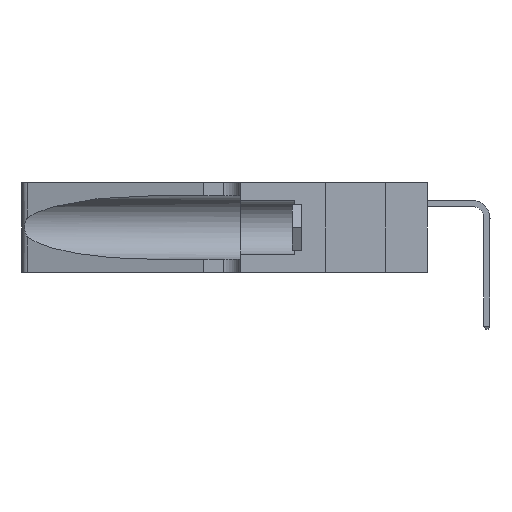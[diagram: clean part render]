
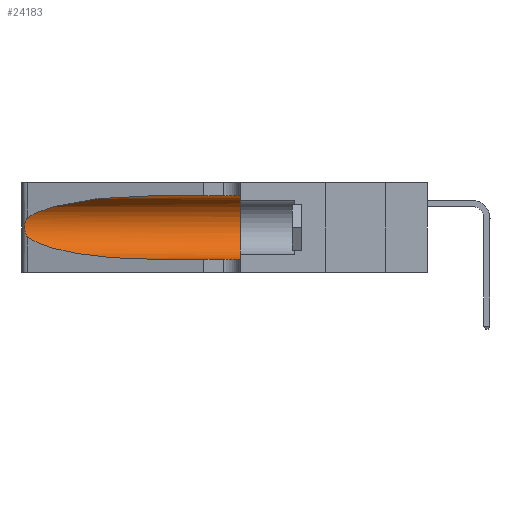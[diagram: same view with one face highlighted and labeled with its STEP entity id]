
A CAD part, left-side view. The second image highlights one B-rep face of the part: STEP entity #24183.
In plain terms, the highlighted cylindrical face has radius 3.308 mm (diameter 6.617 mm), a partial arc.
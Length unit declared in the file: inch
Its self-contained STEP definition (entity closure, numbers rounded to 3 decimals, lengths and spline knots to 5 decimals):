
#430 = CARTESIAN_POINT ( 'NONE',  ( 0.25787, 1.23484, 0.2124 ) ) ;
#478 = CARTESIAN_POINT ( 'NONE',  ( 0.25854, 1.2359, 0.20912 ) ) ;
#664 = CARTESIAN_POINT ( 'NONE',  ( 0.25639, 1.23184, 0.21858 ) ) ;
#1391 = EDGE_LOOP ( 'NONE', ( #30946, #7297, #7504, #7036, #8586, #23628 ) ) ;
#3697 = VERTEX_POINT ( 'NONE', #26931 ) ;
#4834 = EDGE_CURVE ( 'NONE', #18906, #3697, #22312, .T. ) ;
#5140 = CARTESIAN_POINT ( 'NONE',  ( 0.26018, 1.23835, 0.19895 ) ) ;
#5648 = EDGE_CURVE ( 'NONE', #36253, #10619, #7932, .T. ) ;
#7036 = ORIENTED_EDGE ( 'NONE', *, *, #29105, .T. ) ;
#7297 = ORIENTED_EDGE ( 'NONE', *, *, #25240, .T. ) ;
#7504 = ORIENTED_EDGE ( 'NONE', *, *, #5648, .T. ) ;
#7932 =( BOUNDED_CURVE ( )  B_SPLINE_CURVE ( 3, ( #16820, #29108, #18029, #36626 ),
 .UNSPECIFIED., .F., .T. ) 
 B_SPLINE_CURVE_WITH_KNOTS ( ( 4, 4 ),
 ( 3.44316, 4.71239 ),
 .UNSPECIFIED. ) 
 CURVE ( )  GEOMETRIC_REPRESENTATION_ITEM ( )  RATIONAL_B_SPLINE_CURVE ( ( 1., 0.87, 0.87, 1. ) ) 
 REPRESENTATION_ITEM ( '' )  );
#8586 = ORIENTED_EDGE ( 'NONE', *, *, #4834, .F. ) ;
#8799 = CARTESIAN_POINT ( 'NONE',  ( 0.25487, 1.22718, 0.14631 ) ) ;
#9832 = AXIS2_PLACEMENT_3D ( 'NONE', #17270, #25942, #23072 ) ;
#10583 = CARTESIAN_POINT ( 'NONE',  ( 0.1305, 0.72297, 0.31525 ) ) ;
#10619 = VERTEX_POINT ( 'NONE', #29680 ) ;
#10763 = CARTESIAN_POINT ( 'NONE',  ( 0.1305, 1.61858, 0.31525 ) ) ;
#12859 = CARTESIAN_POINT ( 'NONE',  ( 0.25487, 1.22718, 0.22369 ) ) ;
#12988 = CARTESIAN_POINT ( 'NONE',  ( 0.2373, 1.15595, 0.28018 ) ) ;
#13451 = LINE ( 'NONE', #10763, #23285 ) ;
#13997 =( BOUNDED_CURVE ( )  B_SPLINE_CURVE ( 3, ( #24411, #27498, #12988, #33497 ),
 .UNSPECIFIED., .F., .T. ) 
 B_SPLINE_CURVE_WITH_KNOTS ( ( 4, 4 ),
 ( 1.5708, 2.84003 ),
 .UNSPECIFIED. ) 
 CURVE ( )  GEOMETRIC_REPRESENTATION_ITEM ( )  RATIONAL_B_SPLINE_CURVE ( ( 1., 0.87, 0.87, 1. ) ) 
 REPRESENTATION_ITEM ( '' )  );
#14164 = FACE_OUTER_BOUND ( 'NONE', #1391, .T. ) ;
#14249 = VERTEX_POINT ( 'NONE', #10583 ) ;
#15448 = CYLINDRICAL_SURFACE ( 'NONE', #9832, 0.13025 ) ;
#16820 = CARTESIAN_POINT ( 'NONE',  ( 0.25487, 1.22718, 0.14631 ) ) ;
#17270 = CARTESIAN_POINT ( 'NONE',  ( 0.1305, 1.61858, 0.185 ) ) ;
#17485 = VECTOR ( 'NONE', #26968, 39.37008 ) ;
#17696 = LINE ( 'NONE', #24034, #17485 ) ;
#17855 = EDGE_CURVE ( 'NONE', #14249, #18906, #13451, .T. ) ;
#18029 = CARTESIAN_POINT ( 'NONE',  ( 0.18966, 0.96281, 0.05475 ) ) ;
#18906 = VERTEX_POINT ( 'NONE', #31943 ) ;
#19440 = DIRECTION ( 'NONE',  ( 0., -1., 0. ) ) ;
#20241 = VERTEX_POINT ( 'NONE', #12859 ) ;
#22207 = CARTESIAN_POINT ( 'NONE',  ( 0.1305, 0.35, 0.185 ) ) ;
#22312 = CIRCLE ( 'NONE', #26788, 0.13025 ) ;
#23072 = DIRECTION ( 'NONE',  ( 0., 0., -1. ) ) ;
#23285 = VECTOR ( 'NONE', #19440, 39.37008 ) ;
#23628 = ORIENTED_EDGE ( 'NONE', *, *, #17855, .F. ) ;
#24034 = CARTESIAN_POINT ( 'NONE',  ( 0.1305, 1.61858, 0.05475 ) ) ;
#24183 = ADVANCED_FACE ( 'NONE', ( #14164 ), #15448, .F. ) ;
#24411 = CARTESIAN_POINT ( 'NONE',  ( 0.1305, 0.72297, 0.31525 ) ) ;
#25240 = EDGE_CURVE ( 'NONE', #20241, #36253, #27399, .T. ) ;
#25670 = DIRECTION ( 'NONE',  ( 0., 0., 1. ) ) ;
#25942 = DIRECTION ( 'NONE',  ( 0., -1., 0. ) ) ;
#26788 = AXIS2_PLACEMENT_3D ( 'NONE', #22207, #36296, #25670 ) ;
#26931 = CARTESIAN_POINT ( 'NONE',  ( 0.1305, 0.35, 0.05475 ) ) ;
#26968 = DIRECTION ( 'NONE',  ( 0., -1., 0. ) ) ;
#27399 = B_SPLINE_CURVE_WITH_KNOTS ( 'NONE', 3,
 ( #37388, #37234, #664, #430, #478, #5140, #27731, #27726, #27646, #28073, #28239, #28335, #27817, #27683 ),
 .UNSPECIFIED., .F., .F.,
 ( 4, 2, 2, 2, 2, 2, 4 ),
 ( 0., 0.00027, 0.00053, 0.00107, 0.0016, 0.00187, 0.00214 ),
 .UNSPECIFIED. ) ;
#27498 = CARTESIAN_POINT ( 'NONE',  ( 0.18966, 0.96281, 0.31525 ) ) ;
#27646 = CARTESIAN_POINT ( 'NONE',  ( 0.26017, 1.23833, 0.17102 ) ) ;
#27683 = CARTESIAN_POINT ( 'NONE',  ( 0.25487, 1.22718, 0.14631 ) ) ;
#27726 = CARTESIAN_POINT ( 'NONE',  ( 0.26075, 1.23896, 0.178 ) ) ;
#27731 = CARTESIAN_POINT ( 'NONE',  ( 0.26075, 1.23896, 0.19203 ) ) ;
#27817 = CARTESIAN_POINT ( 'NONE',  ( 0.25555, 1.22993, 0.14849 ) ) ;
#28073 = CARTESIAN_POINT ( 'NONE',  ( 0.25856, 1.23593, 0.16098 ) ) ;
#28239 = CARTESIAN_POINT ( 'NONE',  ( 0.25789, 1.23486, 0.15765 ) ) ;
#28335 = CARTESIAN_POINT ( 'NONE',  ( 0.25639, 1.23186, 0.15144 ) ) ;
#29105 = EDGE_CURVE ( 'NONE', #10619, #3697, #17696, .T. ) ;
#29108 = CARTESIAN_POINT ( 'NONE',  ( 0.2373, 1.15595, 0.08982 ) ) ;
#29680 = CARTESIAN_POINT ( 'NONE',  ( 0.1305, 0.72297, 0.05475 ) ) ;
#30946 = ORIENTED_EDGE ( 'NONE', *, *, #36550, .T. ) ;
#31943 = CARTESIAN_POINT ( 'NONE',  ( 0.1305, 0.35, 0.31525 ) ) ;
#33497 = CARTESIAN_POINT ( 'NONE',  ( 0.25487, 1.22718, 0.22369 ) ) ;
#36253 = VERTEX_POINT ( 'NONE', #8799 ) ;
#36296 = DIRECTION ( 'NONE',  ( 0., 1., 0. ) ) ;
#36550 = EDGE_CURVE ( 'NONE', #14249, #20241, #13997, .T. ) ;
#36626 = CARTESIAN_POINT ( 'NONE',  ( 0.1305, 0.72297, 0.05475 ) ) ;
#37234 = CARTESIAN_POINT ( 'NONE',  ( 0.25555, 1.22994, 0.2215 ) ) ;
#37388 = CARTESIAN_POINT ( 'NONE',  ( 0.25487, 1.22718, 0.22369 ) ) ;
